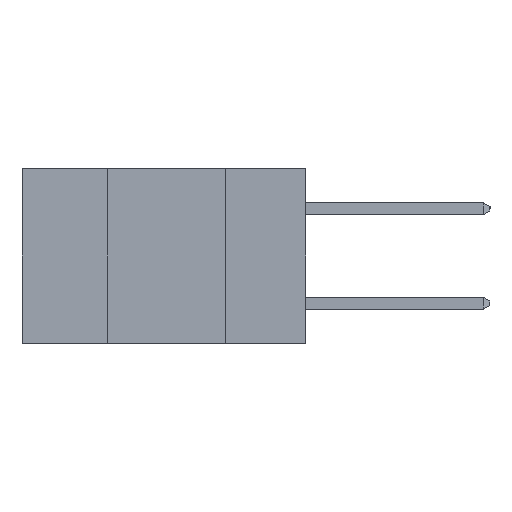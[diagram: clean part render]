
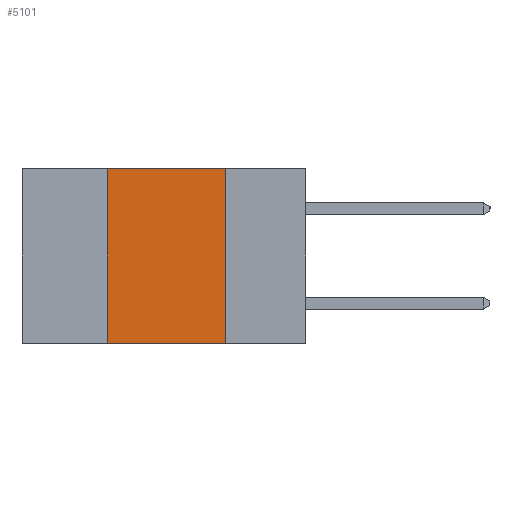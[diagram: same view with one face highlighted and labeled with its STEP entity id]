
A CAD part, left-side view. The second image highlights one B-rep face of the part: STEP entity #5101.
In plain terms, the highlighted planar face has unit normal (-1, 0, 0).
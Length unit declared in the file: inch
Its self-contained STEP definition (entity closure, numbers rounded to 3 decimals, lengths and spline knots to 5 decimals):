
#2 = VERTEX_POINT ( 'NONE', #1521 ) ;
#22 = AXIS2_PLACEMENT_3D ( 'NONE', #5390, #10217, #5140 ) ;
#42 = ORIENTED_EDGE ( 'NONE', *, *, #9999, .F. ) ;
#860 = ORIENTED_EDGE ( 'NONE', *, *, #1064, .T. ) ;
#1064 = EDGE_CURVE ( 'NONE', #2, #6293, #9630, .T. ) ;
#1088 = FACE_OUTER_BOUND ( 'NONE', #6532, .T. ) ;
#1521 = CARTESIAN_POINT ( 'NONE',  ( 0., 0.42, -0.37 ) ) ;
#2821 = CARTESIAN_POINT ( 'NONE',  ( 0., 0.42, 0. ) ) ;
#2958 = VECTOR ( 'NONE', #7742, 39.37008 ) ;
#3271 = DIRECTION ( 'NONE',  ( 0., 0., 1. ) ) ;
#3331 = VECTOR ( 'NONE', #8623, 39.37008 ) ;
#3878 = CARTESIAN_POINT ( 'NONE',  ( 0., 0.6, -0.37 ) ) ;
#4114 = EDGE_CURVE ( 'NONE', #2, #4344, #8946, .T. ) ;
#4344 = VERTEX_POINT ( 'NONE', #2821 ) ;
#4633 = VERTEX_POINT ( 'NONE', #8746 ) ;
#4706 = CARTESIAN_POINT ( 'NONE',  ( 0., 0.17, -0.37 ) ) ;
#4956 = PLANE ( 'NONE',  #22 ) ;
#5101 = ADVANCED_FACE ( 'NONE', ( #1088 ), #4956, .F. ) ;
#5140 = DIRECTION ( 'NONE',  ( 0., 0., -1. ) ) ;
#5141 = ORIENTED_EDGE ( 'NONE', *, *, #7331, .F. ) ;
#5390 = CARTESIAN_POINT ( 'NONE',  ( 0., 0.6, 0. ) ) ;
#6102 = CARTESIAN_POINT ( 'NONE',  ( 0., 0.42, -0.37 ) ) ;
#6293 = VERTEX_POINT ( 'NONE', #4706 ) ;
#6532 = EDGE_LOOP ( 'NONE', ( #5141, #42, #11600, #860 ) ) ;
#7095 = VECTOR ( 'NONE', #3271, 39.37008 ) ;
#7331 = EDGE_CURVE ( 'NONE', #4633, #6293, #8649, .T. ) ;
#7704 = DIRECTION ( 'NONE',  ( 0., 0., -1. ) ) ;
#7742 = DIRECTION ( 'NONE',  ( 0., -1., 0. ) ) ;
#7952 = CARTESIAN_POINT ( 'NONE',  ( 0., 0.17, -0.37 ) ) ;
#8623 = DIRECTION ( 'NONE',  ( 0., -1., 0. ) ) ;
#8649 = LINE ( 'NONE', #7952, #9537 ) ;
#8746 = CARTESIAN_POINT ( 'NONE',  ( 0., 0.17, 0. ) ) ;
#8946 = LINE ( 'NONE', #6102, #7095 ) ;
#9537 = VECTOR ( 'NONE', #7704, 39.37008 ) ;
#9630 = LINE ( 'NONE', #3878, #2958 ) ;
#9999 = EDGE_CURVE ( 'NONE', #4344, #4633, #10366, .T. ) ;
#10217 = DIRECTION ( 'NONE',  ( 1., 0., 0. ) ) ;
#10366 = LINE ( 'NONE', #11245, #3331 ) ;
#11245 = CARTESIAN_POINT ( 'NONE',  ( 0., 0.6, 0. ) ) ;
#11600 = ORIENTED_EDGE ( 'NONE', *, *, #4114, .F. ) ;
